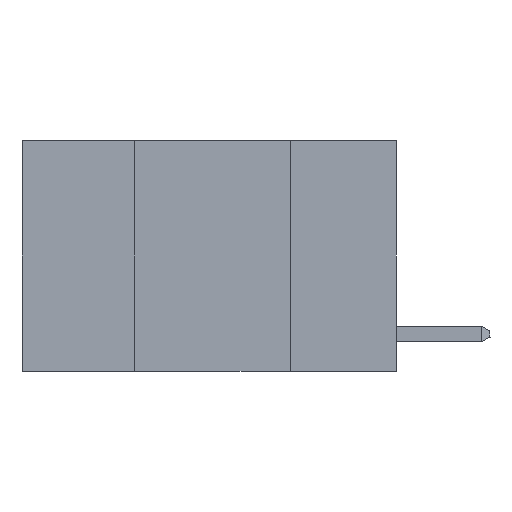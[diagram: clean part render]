
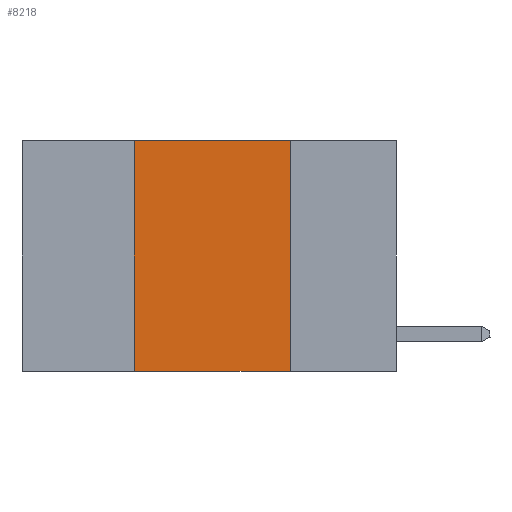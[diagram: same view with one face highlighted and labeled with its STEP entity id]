
A CAD part, left-side view. The second image highlights one B-rep face of the part: STEP entity #8218.
In plain terms, the highlighted planar face has unit normal (-1, 0, 0).
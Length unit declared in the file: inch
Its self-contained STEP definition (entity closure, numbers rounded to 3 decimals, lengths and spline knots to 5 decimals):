
#334 = AXIS2_PLACEMENT_3D ( 'NONE', #10064, #3798, #4718 ) ;
#487 = ORIENTED_EDGE ( 'NONE', *, *, #5093, .T. ) ;
#645 = CARTESIAN_POINT ( 'NONE',  ( 0., 0.6, 0. ) ) ;
#1159 = FACE_OUTER_BOUND ( 'NONE', #8080, .T. ) ;
#1360 = DIRECTION ( 'NONE',  ( 0., 0., -1. ) ) ;
#1613 = VECTOR ( 'NONE', #2620, 39.37008 ) ;
#1734 = CARTESIAN_POINT ( 'NONE',  ( 0., 0.17, 0. ) ) ;
#1983 = DIRECTION ( 'NONE',  ( 0., -1., 0. ) ) ;
#2043 = PLANE ( 'NONE',  #334 ) ;
#2133 = VERTEX_POINT ( 'NONE', #1734 ) ;
#2175 = ORIENTED_EDGE ( 'NONE', *, *, #10938, .F. ) ;
#2246 = DIRECTION ( 'NONE',  ( 0., -1., 0. ) ) ;
#2562 = CARTESIAN_POINT ( 'NONE',  ( 0., 0.42, 0. ) ) ;
#2586 = VERTEX_POINT ( 'NONE', #3902 ) ;
#2620 = DIRECTION ( 'NONE',  ( 0., 0., 1. ) ) ;
#3047 = CARTESIAN_POINT ( 'NONE',  ( 0., 0.42, 0. ) ) ;
#3092 = VECTOR ( 'NONE', #1983, 39.37008 ) ;
#3584 = EDGE_CURVE ( 'NONE', #6854, #2133, #4972, .T. ) ;
#3798 = DIRECTION ( 'NONE',  ( 1., 0., 0. ) ) ;
#3902 = CARTESIAN_POINT ( 'NONE',  ( 0., 0.17, -0.37 ) ) ;
#4049 = VECTOR ( 'NONE', #2246, 39.37008 ) ;
#4270 = CARTESIAN_POINT ( 'NONE',  ( 0., 0.17, 0. ) ) ;
#4324 = ORIENTED_EDGE ( 'NONE', *, *, #3584, .F. ) ;
#4718 = DIRECTION ( 'NONE',  ( 0., 0., -1. ) ) ;
#4972 = LINE ( 'NONE', #645, #4049 ) ;
#5093 = EDGE_CURVE ( 'NONE', #10393, #2586, #7298, .T. ) ;
#5537 = CARTESIAN_POINT ( 'NONE',  ( 0., 0.6, -0.37 ) ) ;
#5942 = VECTOR ( 'NONE', #1360, 39.37008 ) ;
#6854 = VERTEX_POINT ( 'NONE', #3047 ) ;
#7084 = EDGE_CURVE ( 'NONE', #10393, #6854, #8117, .T. ) ;
#7298 = LINE ( 'NONE', #5537, #3092 ) ;
#7328 = ORIENTED_EDGE ( 'NONE', *, *, #7084, .F. ) ;
#7439 = CARTESIAN_POINT ( 'NONE',  ( 0., 0.42, -0.37 ) ) ;
#8080 = EDGE_LOOP ( 'NONE', ( #2175, #4324, #7328, #487 ) ) ;
#8117 = LINE ( 'NONE', #2562, #1613 ) ;
#8218 = ADVANCED_FACE ( 'NONE', ( #1159 ), #2043, .F. ) ;
#10064 = CARTESIAN_POINT ( 'NONE',  ( 0., 0.6, 0. ) ) ;
#10326 = LINE ( 'NONE', #4270, #5942 ) ;
#10393 = VERTEX_POINT ( 'NONE', #7439 ) ;
#10938 = EDGE_CURVE ( 'NONE', #2133, #2586, #10326, .T. ) ;
